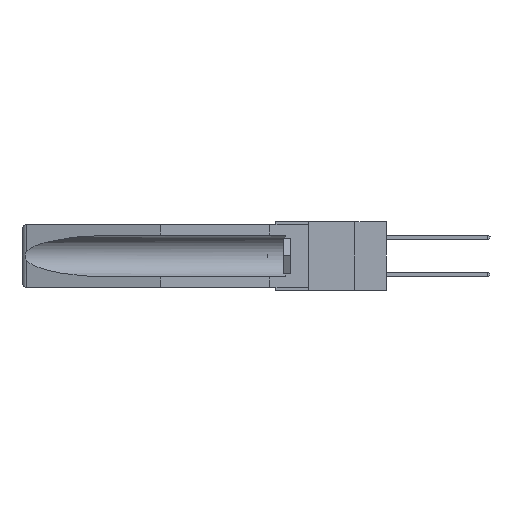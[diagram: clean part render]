
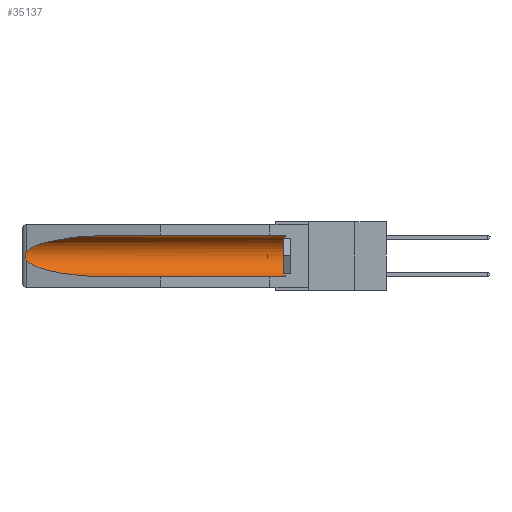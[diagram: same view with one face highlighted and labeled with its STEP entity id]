
A CAD part, left-side view. The second image highlights one B-rep face of the part: STEP entity #35137.
In plain terms, the highlighted cylindrical face has radius 2.857 mm (diameter 5.715 mm), a partial arc.
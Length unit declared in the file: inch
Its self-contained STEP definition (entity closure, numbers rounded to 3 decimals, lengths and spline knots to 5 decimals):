
#778 = CARTESIAN_POINT ( 'NONE',  ( 0.26537, 1.52718, -0.14972 ) ) ;
#1590 = CARTESIAN_POINT ( 'NONE',  ( 0.26597, 1.52961, -0.15275 ) ) ;
#1752 = DIRECTION ( 'NONE',  ( 0., 0., 1. ) ) ;
#2066 = CARTESIAN_POINT ( 'NONE',  ( 0.26537, 1.52718, -0.14972 ) ) ;
#2429 = CARTESIAN_POINT ( 'NONE',  ( 0.26654, 1.53092, -0.15636 ) ) ;
#3035 = VERTEX_POINT ( 'NONE', #8415 ) ;
#3220 = ORIENTED_EDGE ( 'NONE', *, *, #33406, .T. ) ;
#4428 = CARTESIAN_POINT ( 'NONE',  ( 0.21114, 1.30732, -0.284 ) ) ;
#4811 = EDGE_LOOP ( 'NONE', ( #3220, #31499, #9040, #5429, #32750, #34075 ) ) ;
#5429 = ORIENTED_EDGE ( 'NONE', *, *, #20956, .F. ) ;
#5891 = CARTESIAN_POINT ( 'NONE',  ( 0.155, -0.30754, -0.1715 ) ) ;
#6511 = CARTESIAN_POINT ( 'NONE',  ( 0.26537, 1.52718, -0.14972 ) ) ;
#8097 = AXIS2_PLACEMENT_3D ( 'NONE', #30144, #13611, #16430 ) ;
#8415 = CARTESIAN_POINT ( 'NONE',  ( 0.155, 1.07973, -0.284 ) ) ;
#9040 = ORIENTED_EDGE ( 'NONE', *, *, #16019, .T. ) ;
#9042 = CARTESIAN_POINT ( 'NONE',  ( 0.155, 1.07973, -0.059 ) ) ;
#10107 = VERTEX_POINT ( 'NONE', #11104 ) ;
#10333 = FACE_OUTER_BOUND ( 'NONE', #4811, .T. ) ;
#11104 = CARTESIAN_POINT ( 'NONE',  ( 0.155, 0.126, -0.059 ) ) ;
#11175 = DIRECTION ( 'NONE',  ( 0., 1., 0. ) ) ;
#11694 = DIRECTION ( 'NONE',  ( 0., 1., 0. ) ) ;
#11848 = VERTEX_POINT ( 'NONE', #21797 ) ;
#12599 = EDGE_CURVE ( 'NONE', #10107, #28469, #27315, .T. ) ;
#13048 = CARTESIAN_POINT ( 'NONE',  ( 0.25451, 1.48313, -0.24835 ) ) ;
#13611 = DIRECTION ( 'NONE',  ( 0., -1., 0. ) ) ;
#13616 = LINE ( 'NONE', #19553, #15360 ) ;
#14603 = CARTESIAN_POINT ( 'NONE',  ( 0.25451, 1.48313, -0.09465 ) ) ;
#15360 = VECTOR ( 'NONE', #11175, 39.37008 ) ;
#15473 = CARTESIAN_POINT ( 'NONE',  ( 0.155, 1.07973, -0.284 ) ) ;
#16019 = EDGE_CURVE ( 'NONE', #28272, #3035, #33531, .T. ) ;
#16047 = CARTESIAN_POINT ( 'NONE',  ( 0.26537, 1.52718, -0.19328 ) ) ;
#16430 = DIRECTION ( 'NONE',  ( 0., 0., 1. ) ) ;
#19183 = CARTESIAN_POINT ( 'NONE',  ( 0.26597, 1.5296, -0.19026 ) ) ;
#19307 = CARTESIAN_POINT ( 'NONE',  ( 0.2673, 1.5327, -0.16383 ) ) ;
#19553 = CARTESIAN_POINT ( 'NONE',  ( 0.155, -0.30754, -0.284 ) ) ;
#19741 = AXIS2_PLACEMENT_3D ( 'NONE', #5891, #11694, #1752 ) ;
#20956 = EDGE_CURVE ( 'NONE', #11848, #3035, #13616, .T. ) ;
#21046 = CARTESIAN_POINT ( 'NONE',  ( 0.26537, 1.52718, -0.19328 ) ) ;
#21155 = B_SPLINE_CURVE_WITH_KNOTS ( 'NONE', 3,
 ( #2066, #1590, #2429, #19307, #32678, #29773, #24342, #35826, #19183, #16047 ),
 .UNSPECIFIED., .F., .F.,
 ( 4, 2, 2, 2, 4 ),
 ( 0., 0.00029, 0.00058, 0.00087, 0.00117 ),
 .UNSPECIFIED. ) ;
#21797 = CARTESIAN_POINT ( 'NONE',  ( 0.155, 0.126, -0.284 ) ) ;
#21868 = CARTESIAN_POINT ( 'NONE',  ( 0.155, -0.30754, -0.059 ) ) ;
#22535 = CARTESIAN_POINT ( 'NONE',  ( 0.155, 1.07973, -0.059 ) ) ;
#23200 = EDGE_CURVE ( 'NONE', #11848, #10107, #28563, .T. ) ;
#24342 = CARTESIAN_POINT ( 'NONE',  ( 0.2673, 1.53269, -0.17917 ) ) ;
#25222 = CARTESIAN_POINT ( 'NONE',  ( 0.21114, 1.30732, -0.059 ) ) ;
#25604 = DIRECTION ( 'NONE',  ( 0., 1., 0. ) ) ;
#26677 = VERTEX_POINT ( 'NONE', #6511 ) ;
#27315 = LINE ( 'NONE', #21868, #29463 ) ;
#27574 = CYLINDRICAL_SURFACE ( 'NONE', #19741, 0.1125 ) ;
#28272 = VERTEX_POINT ( 'NONE', #34553 ) ;
#28469 = VERTEX_POINT ( 'NONE', #22535 ) ;
#28563 = CIRCLE ( 'NONE', #8097, 0.1125 ) ;
#29463 = VECTOR ( 'NONE', #25604, 39.37008 ) ;
#29773 = CARTESIAN_POINT ( 'NONE',  ( 0.2675, 1.53308, -0.17534 ) ) ;
#30144 = CARTESIAN_POINT ( 'NONE',  ( 0.155, 0.126, -0.1715 ) ) ;
#31499 = ORIENTED_EDGE ( 'NONE', *, *, #33792, .T. ) ;
#32678 = CARTESIAN_POINT ( 'NONE',  ( 0.2675, 1.53308, -0.16763 ) ) ;
#32750 = ORIENTED_EDGE ( 'NONE', *, *, #23200, .T. ) ;
#33059 =( BOUNDED_CURVE ( )  B_SPLINE_CURVE ( 3, ( #9042, #25222, #14603, #778 ),
 .UNSPECIFIED., .F., .F. ) 
 B_SPLINE_CURVE_WITH_KNOTS ( ( 4, 4 ),
 ( 4.71239, 6.08839 ),
 .UNSPECIFIED. ) 
 CURVE ( )  GEOMETRIC_REPRESENTATION_ITEM ( )  RATIONAL_B_SPLINE_CURVE ( ( 1., 0.848, 0.848, 1. ) ) 
 REPRESENTATION_ITEM ( '' )  );
#33406 = EDGE_CURVE ( 'NONE', #28469, #26677, #33059, .T. ) ;
#33531 =( BOUNDED_CURVE ( )  B_SPLINE_CURVE ( 3, ( #21046, #13048, #4428, #15473 ),
 .UNSPECIFIED., .F., .F. ) 
 B_SPLINE_CURVE_WITH_KNOTS ( ( 4, 4 ),
 ( 0.1948, 1.5708 ),
 .UNSPECIFIED. ) 
 CURVE ( )  GEOMETRIC_REPRESENTATION_ITEM ( )  RATIONAL_B_SPLINE_CURVE ( ( 1., 0.848, 0.848, 1. ) ) 
 REPRESENTATION_ITEM ( '' )  );
#33792 = EDGE_CURVE ( 'NONE', #26677, #28272, #21155, .T. ) ;
#34075 = ORIENTED_EDGE ( 'NONE', *, *, #12599, .T. ) ;
#34553 = CARTESIAN_POINT ( 'NONE',  ( 0.26537, 1.52718, -0.19328 ) ) ;
#35137 = ADVANCED_FACE ( 'NONE', ( #10333 ), #27574, .F. ) ;
#35826 = CARTESIAN_POINT ( 'NONE',  ( 0.26655, 1.53094, -0.18657 ) ) ;
